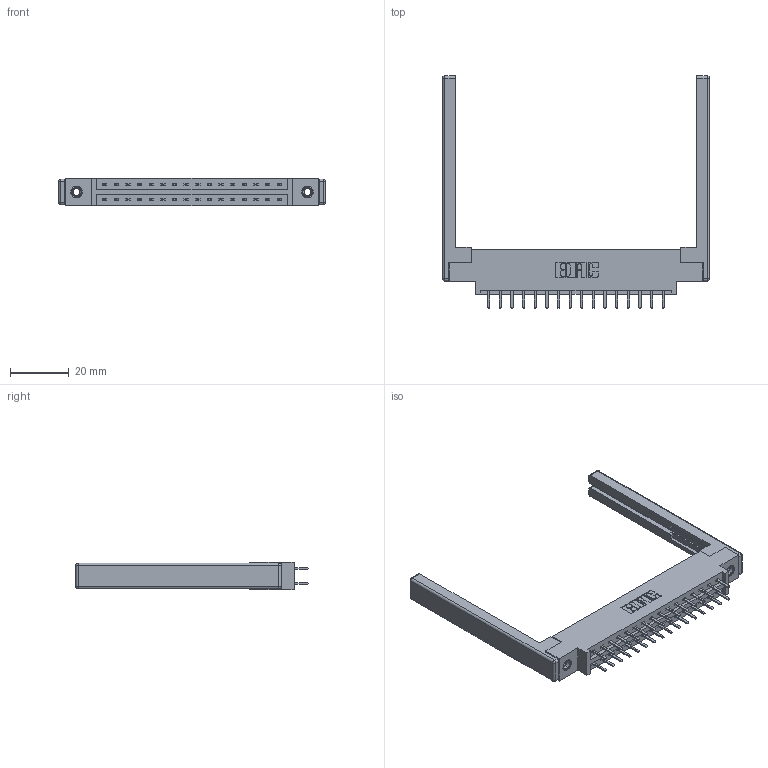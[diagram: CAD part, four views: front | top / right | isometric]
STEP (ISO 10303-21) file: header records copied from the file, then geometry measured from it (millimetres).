
FILE_DESCRIPTION (( 'STEP AP203' ), '1' );
FILE_NAME ('337-032-520-868.STEP', '2019-10-11T00:28:57', ( '' ), ( '' ), 'SwSTEP 2.0', 'SolidWorks 2016', '' );
FILE_SCHEMA (( 'CONFIG_CONTROL_DESIGN' ));
Length unit declared in the file: inch
Products named in the file (5): 337 Part_0.170 Offset - 0.156 Dia-TI; 337-032-520-868; 345-292-001_345-293-120; 307-220-068; 345-250-001_345-250-001-102
Assembly tree (37 placements, depth 2):
  337-032-520-868
    337 Part_0.170 Offset - 0.156 Dia-TI
    345-292-001_345-293-120  x32
    345-250-001_345-250-001-102  x2
    307-220-068  x2
Bounding box: 90.83 x 79.08 x 9.4 mm (x, y, z)
Volume: 13479.6 mm3; surface area: 14131.2 mm2
Topology: 37 solids, 37 shells, 2128 faces, 6121 edges, 3974 vertices
Faces by surface type: plane 1442, cylinder 662, cone 12, sphere 8, torus 4
Entity records: 18774 total; most frequent: CARTESIAN_POINT 3163, ORIENTED_EDGE 3076, DIRECTION 2796, EDGE_CURVE 1538, VECTOR 1356, LINE 1356, VERTEX_POINT 1014, AXIS2_PLACEMENT_3D 720
